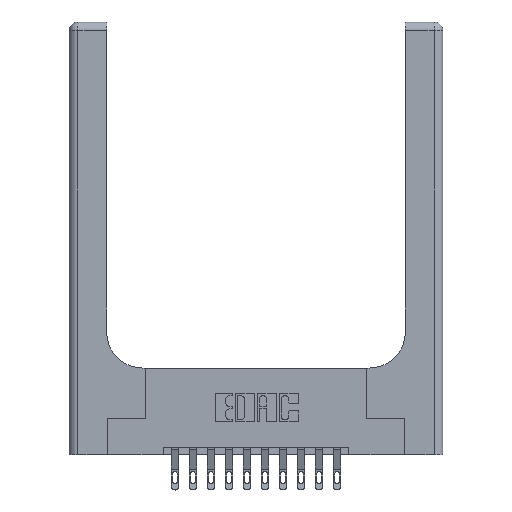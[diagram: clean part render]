
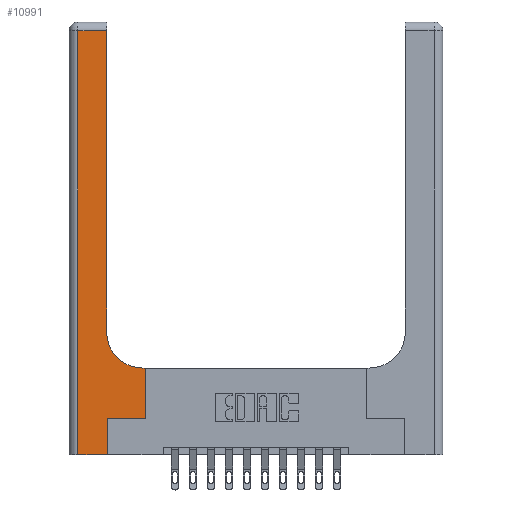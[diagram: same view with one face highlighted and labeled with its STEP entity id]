
A CAD part, top view. The second image highlights one B-rep face of the part: STEP entity #10991.
In plain terms, the highlighted planar face has unit normal (0, 0, 1).
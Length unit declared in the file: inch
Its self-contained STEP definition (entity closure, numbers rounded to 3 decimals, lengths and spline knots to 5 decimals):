
#286 = VECTOR ( 'NONE', #9677, 39.37008 ) ;
#615 = ORIENTED_EDGE ( 'NONE', *, *, #16034, .T. ) ;
#869 = DIRECTION ( 'NONE',  ( -1., 0., 0. ) ) ;
#1193 = EDGE_CURVE ( 'NONE', #11827, #3845, #4474, .T. ) ;
#1331 = DIRECTION ( 'NONE',  ( 0., 1., 0. ) ) ;
#1494 = LINE ( 'NONE', #7784, #14569 ) ;
#1514 = CARTESIAN_POINT ( 'NONE',  ( 0.528, 0.25, 0.37 ) ) ;
#1595 = ORIENTED_EDGE ( 'NONE', *, *, #15233, .T. ) ;
#1615 = VECTOR ( 'NONE', #14645, 39.37008 ) ;
#1702 = DIRECTION ( 'NONE',  ( -1., 0., 0. ) ) ;
#1929 = ORIENTED_EDGE ( 'NONE', *, *, #13475, .T. ) ;
#2775 = CARTESIAN_POINT ( 'NONE',  ( 0.51, 0.85, 0.37 ) ) ;
#2795 = ORIENTED_EDGE ( 'NONE', *, *, #1193, .T. ) ;
#2831 = DIRECTION ( 'NONE',  ( 0., 0., -1. ) ) ;
#2941 = LINE ( 'NONE', #10520, #15978 ) ;
#2942 = VERTEX_POINT ( 'NONE', #11064 ) ;
#3255 = AXIS2_PLACEMENT_3D ( 'NONE', #5489, #8244, #13205 ) ;
#3294 = VECTOR ( 'NONE', #869, 39.37008 ) ;
#3845 = VERTEX_POINT ( 'NONE', #6344 ) ;
#4474 = LINE ( 'NONE', #10761, #9192 ) ;
#4498 = EDGE_CURVE ( 'NONE', #7664, #15689, #11843, .T. ) ;
#4679 = VERTEX_POINT ( 'NONE', #14267 ) ;
#5254 = VECTOR ( 'NONE', #7392, 39.37008 ) ;
#5298 = CARTESIAN_POINT ( 'NONE',  ( 0.06, 3., 0.37 ) ) ;
#5309 = EDGE_CURVE ( 'NONE', #15709, #7664, #2941, .T. ) ;
#5489 = CARTESIAN_POINT ( 'NONE',  ( 0., 3., 0.37 ) ) ;
#6072 = LINE ( 'NONE', #12653, #15363 ) ;
#6298 = VERTEX_POINT ( 'NONE', #1514 ) ;
#6344 = CARTESIAN_POINT ( 'NONE',  ( 0.265, 0., 0.37 ) ) ;
#6436 = LINE ( 'NONE', #5298, #5254 ) ;
#6706 = EDGE_CURVE ( 'NONE', #15689, #2942, #6072, .T. ) ;
#7392 = DIRECTION ( 'NONE',  ( 0., -1., 0. ) ) ;
#7393 = ORIENTED_EDGE ( 'NONE', *, *, #11148, .T. ) ;
#7664 = VERTEX_POINT ( 'NONE', #11905 ) ;
#7784 = CARTESIAN_POINT ( 'NONE',  ( 0.265, 0.25, 0.37 ) ) ;
#7835 = DIRECTION ( 'NONE',  ( 1., 0., 0. ) ) ;
#8189 = PLANE ( 'NONE',  #3255 ) ;
#8244 = DIRECTION ( 'NONE',  ( 0., 0., -1. ) ) ;
#8290 = CARTESIAN_POINT ( 'NONE',  ( 0.265, 0., 0.37 ) ) ;
#8296 = ORIENTED_EDGE ( 'NONE', *, *, #5309, .T. ) ;
#9192 = VECTOR ( 'NONE', #9619, 39.37008 ) ;
#9604 = CARTESIAN_POINT ( 'NONE',  ( 0.265, 0.25, 0.37 ) ) ;
#9619 = DIRECTION ( 'NONE',  ( 1., 0., 0. ) ) ;
#9660 = CARTESIAN_POINT ( 'NONE',  ( 0., 2.94, 0.37 ) ) ;
#9677 = DIRECTION ( 'NONE',  ( 0., 1., 0. ) ) ;
#10197 = EDGE_LOOP ( 'NONE', ( #14315, #7393, #15375, #2795, #1929, #1595, #615, #8296, #13473 ) ) ;
#10520 = CARTESIAN_POINT ( 'NONE',  ( 0.26, 0.6, 0.37 ) ) ;
#10761 = CARTESIAN_POINT ( 'NONE',  ( 0., 0., 0.37 ) ) ;
#10991 = ADVANCED_FACE ( 'NONE', ( #15748 ), #8189, .F. ) ;
#11064 = CARTESIAN_POINT ( 'NONE',  ( 0.26, 2.94, 0.37 ) ) ;
#11148 = EDGE_CURVE ( 'NONE', #2942, #4679, #13163, .T. ) ;
#11827 = VERTEX_POINT ( 'NONE', #12462 ) ;
#11843 = CIRCLE ( 'NONE', #15250, 0.25 ) ;
#11905 = CARTESIAN_POINT ( 'NONE',  ( 0.51, 0.6, 0.37 ) ) ;
#12166 = CARTESIAN_POINT ( 'NONE',  ( 0.528, 0.6, 0.37 ) ) ;
#12462 = CARTESIAN_POINT ( 'NONE',  ( 0.06, 0., 0.37 ) ) ;
#12653 = CARTESIAN_POINT ( 'NONE',  ( 0.26, 3., 0.37 ) ) ;
#12863 = DIRECTION ( 'NONE',  ( 1., 0., 0. ) ) ;
#13163 = LINE ( 'NONE', #9660, #3294 ) ;
#13205 = DIRECTION ( 'NONE',  ( -1., 0., 0. ) ) ;
#13390 = CARTESIAN_POINT ( 'NONE',  ( 0.528, 0.25, 0.37 ) ) ;
#13473 = ORIENTED_EDGE ( 'NONE', *, *, #4498, .T. ) ;
#13475 = EDGE_CURVE ( 'NONE', #3845, #13504, #16240, .T. ) ;
#13504 = VERTEX_POINT ( 'NONE', #9604 ) ;
#14267 = CARTESIAN_POINT ( 'NONE',  ( 0.06, 2.94, 0.37 ) ) ;
#14315 = ORIENTED_EDGE ( 'NONE', *, *, #6706, .T. ) ;
#14569 = VECTOR ( 'NONE', #7835, 39.37008 ) ;
#14645 = DIRECTION ( 'NONE',  ( 0., 1., 0. ) ) ;
#15233 = EDGE_CURVE ( 'NONE', #13504, #6298, #1494, .T. ) ;
#15250 = AXIS2_PLACEMENT_3D ( 'NONE', #2775, #2831, #12863 ) ;
#15363 = VECTOR ( 'NONE', #1331, 39.37008 ) ;
#15375 = ORIENTED_EDGE ( 'NONE', *, *, #15380, .T. ) ;
#15380 = EDGE_CURVE ( 'NONE', #4679, #11827, #6436, .T. ) ;
#15689 = VERTEX_POINT ( 'NONE', #16044 ) ;
#15709 = VERTEX_POINT ( 'NONE', #12166 ) ;
#15748 = FACE_OUTER_BOUND ( 'NONE', #10197, .T. ) ;
#15978 = VECTOR ( 'NONE', #1702, 39.37008 ) ;
#16034 = EDGE_CURVE ( 'NONE', #6298, #15709, #16090, .T. ) ;
#16044 = CARTESIAN_POINT ( 'NONE',  ( 0.26, 0.85, 0.37 ) ) ;
#16090 = LINE ( 'NONE', #13390, #286 ) ;
#16240 = LINE ( 'NONE', #8290, #1615 ) ;
